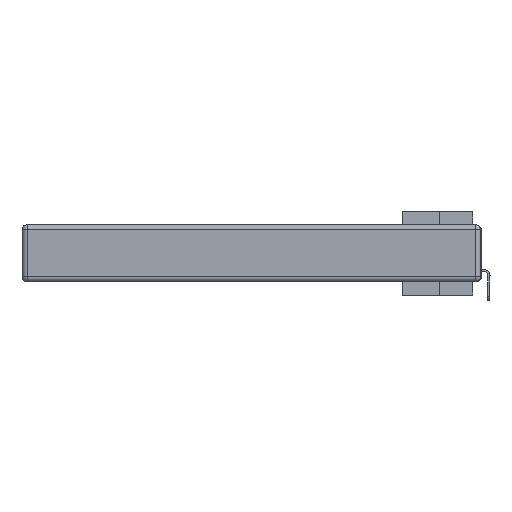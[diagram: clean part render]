
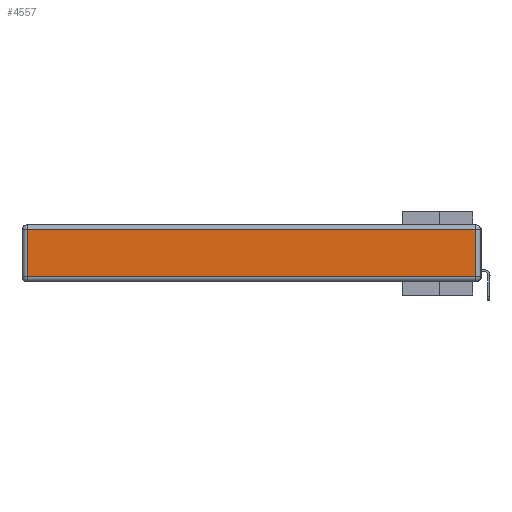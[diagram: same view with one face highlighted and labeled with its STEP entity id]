
A CAD part, left-side view. The second image highlights one B-rep face of the part: STEP entity #4557.
In plain terms, the highlighted planar face has unit normal (-1, 0, 0).
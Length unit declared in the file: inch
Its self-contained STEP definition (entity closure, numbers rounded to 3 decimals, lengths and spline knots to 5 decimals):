
#13 = VERTEX_POINT ( 'NONE', #26457 ) ;
#867 = CARTESIAN_POINT ( 'NONE',  ( 0., 0.03, -0.343 ) ) ;
#1718 = VERTEX_POINT ( 'NONE', #14561 ) ;
#2619 = DIRECTION ( 'NONE',  ( 0., 0., 1. ) ) ;
#2960 = ORIENTED_EDGE ( 'NONE', *, *, #12403, .T. ) ;
#3769 = CARTESIAN_POINT ( 'NONE',  ( 0., 2.72, -0.343 ) ) ;
#4557 = ADVANCED_FACE ( 'NONE', ( #11252 ), #9604, .T. ) ;
#5197 = LINE ( 'NONE', #867, #21223 ) ;
#5252 = VECTOR ( 'NONE', #18363, 39.37008 ) ;
#5327 = VERTEX_POINT ( 'NONE', #18042 ) ;
#5515 = VECTOR ( 'NONE', #9458, 39.37008 ) ;
#5697 = LINE ( 'NONE', #3769, #20642 ) ;
#5726 = EDGE_CURVE ( 'NONE', #5327, #13, #13632, .T. ) ;
#7506 = DIRECTION ( 'NONE',  ( -1., 0., 0. ) ) ;
#8513 = DIRECTION ( 'NONE',  ( 0., 0., -1. ) ) ;
#9458 = DIRECTION ( 'NONE',  ( 0., -1., 0. ) ) ;
#9604 = PLANE ( 'NONE',  #25279 ) ;
#11252 = FACE_OUTER_BOUND ( 'NONE', #16329, .T. ) ;
#12403 = EDGE_CURVE ( 'NONE', #18733, #1718, #15708, .T. ) ;
#13632 = LINE ( 'NONE', #20605, #5515 ) ;
#13988 = ORIENTED_EDGE ( 'NONE', *, *, #5726, .T. ) ;
#14561 = CARTESIAN_POINT ( 'NONE',  ( 0., 2.72, -0.03 ) ) ;
#15708 = LINE ( 'NONE', #26974, #5252 ) ;
#16329 = EDGE_LOOP ( 'NONE', ( #13988, #21093, #2960, #19571 ) ) ;
#17205 = CARTESIAN_POINT ( 'NONE',  ( 0., 0.03, -0.03 ) ) ;
#18042 = CARTESIAN_POINT ( 'NONE',  ( 0., 2.72, -0.313 ) ) ;
#18363 = DIRECTION ( 'NONE',  ( 0., 1., 0. ) ) ;
#18733 = VERTEX_POINT ( 'NONE', #17205 ) ;
#19571 = ORIENTED_EDGE ( 'NONE', *, *, #20052, .T. ) ;
#20052 = EDGE_CURVE ( 'NONE', #1718, #5327, #5697, .T. ) ;
#20605 = CARTESIAN_POINT ( 'NONE',  ( 0., 0., -0.313 ) ) ;
#20642 = VECTOR ( 'NONE', #8513, 39.37008 ) ;
#20745 = CARTESIAN_POINT ( 'NONE',  ( 0., 0., -0.343 ) ) ;
#21093 = ORIENTED_EDGE ( 'NONE', *, *, #21968, .T. ) ;
#21223 = VECTOR ( 'NONE', #21386, 39.37008 ) ;
#21386 = DIRECTION ( 'NONE',  ( 0., 0., 1. ) ) ;
#21968 = EDGE_CURVE ( 'NONE', #13, #18733, #5197, .T. ) ;
#25279 = AXIS2_PLACEMENT_3D ( 'NONE', #20745, #7506, #2619 ) ;
#26457 = CARTESIAN_POINT ( 'NONE',  ( 0., 0.03, -0.313 ) ) ;
#26974 = CARTESIAN_POINT ( 'NONE',  ( 0., 2.75, -0.03 ) ) ;
